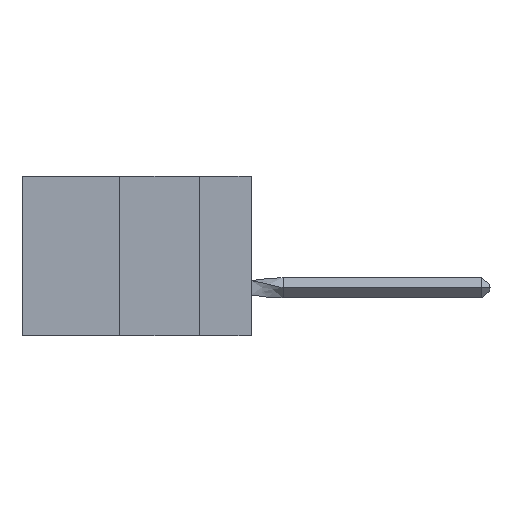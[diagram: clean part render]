
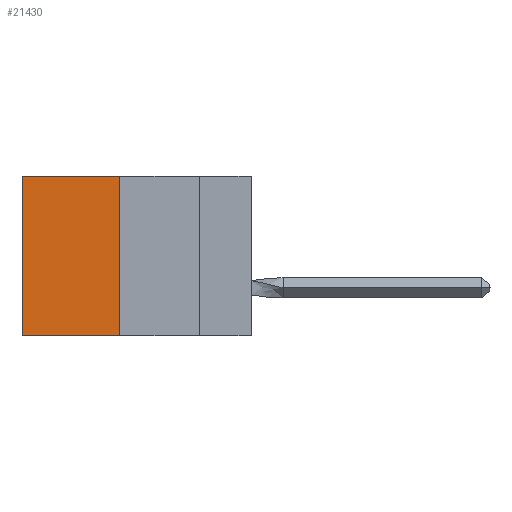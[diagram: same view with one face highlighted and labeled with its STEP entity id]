
A CAD part, left-side view. The second image highlights one B-rep face of the part: STEP entity #21430.
In plain terms, the highlighted planar face has unit normal (-1, 0, 0).
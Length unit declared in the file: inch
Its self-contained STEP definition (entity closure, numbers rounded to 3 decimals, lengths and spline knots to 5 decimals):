
#106 = DIRECTION ( 'NONE',  ( 0., 0., -1. ) ) ;
#422 = ORIENTED_EDGE ( 'NONE', *, *, #3223, .F. ) ;
#595 = DIRECTION ( 'NONE',  ( 0., 0., -1. ) ) ;
#1014 = VECTOR ( 'NONE', #2822, 39.37008 ) ;
#1562 = EDGE_CURVE ( 'NONE', #23126, #14202, #23937, .T. ) ;
#2822 = DIRECTION ( 'NONE',  ( 0., 0., -1. ) ) ;
#2899 = EDGE_CURVE ( 'NONE', #14202, #19782, #3925, .T. ) ;
#3223 = EDGE_CURVE ( 'NONE', #23126, #13114, #22733, .T. ) ;
#3925 = LINE ( 'NONE', #14658, #23021 ) ;
#5524 = CARTESIAN_POINT ( 'NONE',  ( 0.305, 0.413, 0. ) ) ;
#5887 = ORIENTED_EDGE ( 'NONE', *, *, #2899, .T. ) ;
#6742 = CARTESIAN_POINT ( 'NONE',  ( 0.305, 0.413, -0.5 ) ) ;
#7057 = CARTESIAN_POINT ( 'NONE',  ( 0.305, 0.413, -0.5 ) ) ;
#7319 = CARTESIAN_POINT ( 'NONE',  ( 0.305, 0.72, 0. ) ) ;
#9686 = PLANE ( 'NONE',  #18649 ) ;
#10187 = VECTOR ( 'NONE', #18008, 39.37008 ) ;
#10454 = DIRECTION ( 'NONE',  ( 0., 1., 0. ) ) ;
#12694 = ORIENTED_EDGE ( 'NONE', *, *, #1562, .T. ) ;
#13114 = VERTEX_POINT ( 'NONE', #22531 ) ;
#13271 = VECTOR ( 'NONE', #10454, 39.37008 ) ;
#14202 = VERTEX_POINT ( 'NONE', #7319 ) ;
#14658 = CARTESIAN_POINT ( 'NONE',  ( 0.305, 0.72, -0.5 ) ) ;
#14703 = CARTESIAN_POINT ( 'NONE',  ( 0.305, 0.72, -0.5 ) ) ;
#17015 = CARTESIAN_POINT ( 'NONE',  ( 0.305, 0.413, -0.5 ) ) ;
#17361 = LINE ( 'NONE', #7057, #10187 ) ;
#17546 = FACE_OUTER_BOUND ( 'NONE', #17727, .T. ) ;
#17727 = EDGE_LOOP ( 'NONE', ( #5887, #19248, #422, #12694 ) ) ;
#17841 = CARTESIAN_POINT ( 'NONE',  ( 0.305, 0.413, 0. ) ) ;
#18008 = DIRECTION ( 'NONE',  ( 0., 1., 0. ) ) ;
#18649 = AXIS2_PLACEMENT_3D ( 'NONE', #17015, #22685, #595 ) ;
#19248 = ORIENTED_EDGE ( 'NONE', *, *, #19616, .F. ) ;
#19616 = EDGE_CURVE ( 'NONE', #13114, #19782, #17361, .T. ) ;
#19782 = VERTEX_POINT ( 'NONE', #14703 ) ;
#21430 = ADVANCED_FACE ( 'NONE', ( #17546 ), #9686, .F. ) ;
#22531 = CARTESIAN_POINT ( 'NONE',  ( 0.305, 0.413, -0.5 ) ) ;
#22685 = DIRECTION ( 'NONE',  ( 1., 0., 0. ) ) ;
#22733 = LINE ( 'NONE', #6742, #1014 ) ;
#23021 = VECTOR ( 'NONE', #106, 39.37008 ) ;
#23126 = VERTEX_POINT ( 'NONE', #5524 ) ;
#23937 = LINE ( 'NONE', #17841, #13271 ) ;
